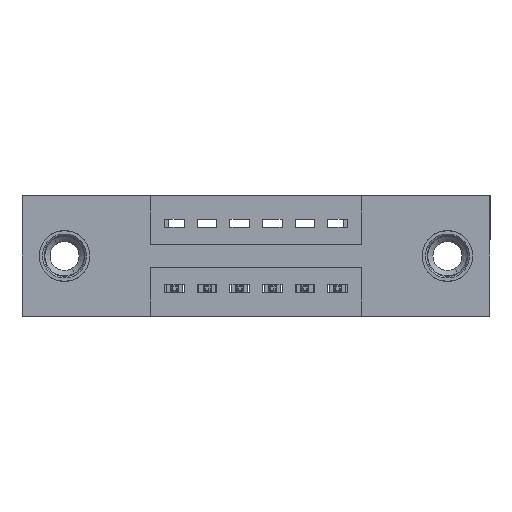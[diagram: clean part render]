
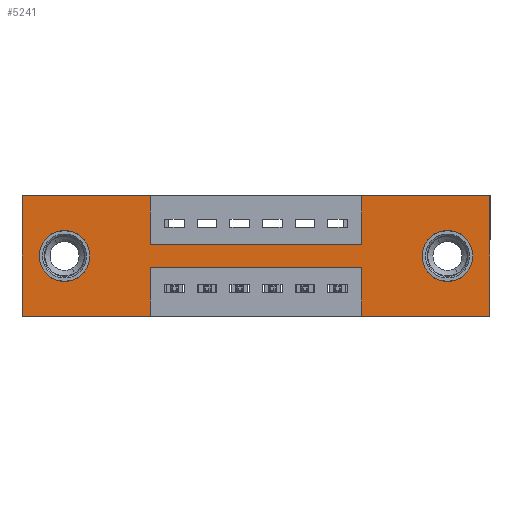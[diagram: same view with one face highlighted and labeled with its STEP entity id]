
A CAD part, front view. The second image highlights one B-rep face of the part: STEP entity #5241.
In plain terms, the highlighted planar face has unit normal (0, -1, 0).
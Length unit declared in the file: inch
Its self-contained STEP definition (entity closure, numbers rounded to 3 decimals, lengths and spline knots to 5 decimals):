
#17 = VECTOR ( 'NONE', #4863, 39.37008 ) ;
#43 = FACE_BOUND ( 'NONE', #11354, .T. ) ;
#104 = CARTESIAN_POINT ( 'NONE',  ( 0., 0., 0. ) ) ;
#146 = LINE ( 'NONE', #10268, #17 ) ;
#180 = FACE_BOUND ( 'NONE', #6715, .T. ) ;
#219 = LINE ( 'NONE', #3082, #7066 ) ;
#233 = CIRCLE ( 'NONE', #9413, 0.078 ) ;
#459 = CARTESIAN_POINT ( 'NONE',  ( 0.3925, 0., -0.37 ) ) ;
#470 = EDGE_CURVE ( 'NONE', #2482, #10637, #7007, .T. ) ;
#523 = ORIENTED_EDGE ( 'NONE', *, *, #9056, .F. ) ;
#635 = DIRECTION ( 'NONE',  ( 0., 0., 1. ) ) ;
#657 = VECTOR ( 'NONE', #8724, 39.37008 ) ;
#661 = EDGE_CURVE ( 'NONE', #3504, #2567, #8666, .T. ) ;
#708 = CARTESIAN_POINT ( 'NONE',  ( 0.13, 0., -0.185 ) ) ;
#1033 = EDGE_CURVE ( 'NONE', #4580, #10286, #233, .T. ) ;
#1054 = ORIENTED_EDGE ( 'NONE', *, *, #7691, .F. ) ;
#1228 = VECTOR ( 'NONE', #2541, 39.37008 ) ;
#1358 = CARTESIAN_POINT ( 'NONE',  ( 1.0425, 0., -0.37 ) ) ;
#1514 = DIRECTION ( 'NONE',  ( 0., 0., 1. ) ) ;
#1562 = EDGE_CURVE ( 'NONE', #10637, #1788, #7770, .T. ) ;
#1593 = VERTEX_POINT ( 'NONE', #459 ) ;
#1699 = EDGE_CURVE ( 'NONE', #10286, #4580, #2029, .T. ) ;
#1788 = VERTEX_POINT ( 'NONE', #7970 ) ;
#1965 = CARTESIAN_POINT ( 'NONE',  ( 0., 0., 0. ) ) ;
#2029 = CIRCLE ( 'NONE', #9501, 0.078 ) ;
#2146 = AXIS2_PLACEMENT_3D ( 'NONE', #708, #7070, #7958 ) ;
#2389 = CARTESIAN_POINT ( 'NONE',  ( 1.0425, 0., -0.37 ) ) ;
#2407 = DIRECTION ( 'NONE',  ( 0., 1., 0. ) ) ;
#2482 = VERTEX_POINT ( 'NONE', #2389 ) ;
#2541 = DIRECTION ( 'NONE',  ( 1., 0., 0. ) ) ;
#2544 = ORIENTED_EDGE ( 'NONE', *, *, #1699, .T. ) ;
#2567 = VERTEX_POINT ( 'NONE', #7847 ) ;
#2642 = VERTEX_POINT ( 'NONE', #10920 ) ;
#2675 = EDGE_CURVE ( 'NONE', #8508, #5809, #8761, .T. ) ;
#2683 = EDGE_CURVE ( 'NONE', #10607, #2482, #9181, .T. ) ;
#2784 = CARTESIAN_POINT ( 'NONE',  ( 0.3925, 0., 0. ) ) ;
#2959 = VERTEX_POINT ( 'NONE', #7315 ) ;
#3060 = LINE ( 'NONE', #6096, #1228 ) ;
#3082 = CARTESIAN_POINT ( 'NONE',  ( 0., 0., -0.37 ) ) ;
#3103 = ORIENTED_EDGE ( 'NONE', *, *, #1562, .F. ) ;
#3242 = VECTOR ( 'NONE', #1514, 39.37008 ) ;
#3504 = VERTEX_POINT ( 'NONE', #9327 ) ;
#3509 = AXIS2_PLACEMENT_3D ( 'NONE', #11296, #5954, #635 ) ;
#3609 = DIRECTION ( 'NONE',  ( 0., 0., -1. ) ) ;
#3691 = EDGE_CURVE ( 'NONE', #10549, #3504, #5065, .T. ) ;
#3826 = VERTEX_POINT ( 'NONE', #5924 ) ;
#4107 = CARTESIAN_POINT ( 'NONE',  ( 0.13, 0., -0.107 ) ) ;
#4234 = PLANE ( 'NONE',  #11470 ) ;
#4265 = ORIENTED_EDGE ( 'NONE', *, *, #4468, .T. ) ;
#4450 = CIRCLE ( 'NONE', #2146, 0.078 ) ;
#4468 = EDGE_CURVE ( 'NONE', #5205, #2642, #8943, .T. ) ;
#4569 = EDGE_CURVE ( 'NONE', #2642, #5205, #4450, .T. ) ;
#4580 = VERTEX_POINT ( 'NONE', #11513 ) ;
#4613 = EDGE_CURVE ( 'NONE', #2959, #3826, #3060, .T. ) ;
#4863 = DIRECTION ( 'NONE',  ( 1., 0., 0. ) ) ;
#5064 = DIRECTION ( 'NONE',  ( 0., -1., 0. ) ) ;
#5065 = LINE ( 'NONE', #2784, #7157 ) ;
#5131 = EDGE_LOOP ( 'NONE', ( #523, #3103, #6701, #5270, #8133, #9442, #1054, #9824, #9307, #5252, #9196, #10583 ) ) ;
#5167 = CARTESIAN_POINT ( 'NONE',  ( 1.0425, 0., 0. ) ) ;
#5205 = VERTEX_POINT ( 'NONE', #4107 ) ;
#5231 = LINE ( 'NONE', #5251, #8160 ) ;
#5241 = ADVANCED_FACE ( 'NONE', ( #43, #180, #6618 ), #4234, .T. ) ;
#5251 = CARTESIAN_POINT ( 'NONE',  ( 0.3925, 0., -0.37 ) ) ;
#5252 = ORIENTED_EDGE ( 'NONE', *, *, #10507, .F. ) ;
#5270 = ORIENTED_EDGE ( 'NONE', *, *, #2683, .F. ) ;
#5283 = DIRECTION ( 'NONE',  ( 0., 0., -1. ) ) ;
#5401 = DIRECTION ( 'NONE',  ( -1., 0., 0. ) ) ;
#5557 = DIRECTION ( 'NONE',  ( 0., 0., 1. ) ) ;
#5809 = VERTEX_POINT ( 'NONE', #1965 ) ;
#5924 = CARTESIAN_POINT ( 'NONE',  ( 1.435, 0., 0. ) ) ;
#5954 = DIRECTION ( 'NONE',  ( 0., 1., 0. ) ) ;
#6096 = CARTESIAN_POINT ( 'NONE',  ( 0., 0., 0. ) ) ;
#6148 = VECTOR ( 'NONE', #9703, 39.37008 ) ;
#6312 = CARTESIAN_POINT ( 'NONE',  ( 0., 0., -0.37 ) ) ;
#6618 = FACE_OUTER_BOUND ( 'NONE', #5131, .T. ) ;
#6655 = VECTOR ( 'NONE', #5401, 39.37008 ) ;
#6701 = ORIENTED_EDGE ( 'NONE', *, *, #470, .F. ) ;
#6715 = EDGE_LOOP ( 'NONE', ( #4265, #6890 ) ) ;
#6769 = ORIENTED_EDGE ( 'NONE', *, *, #1033, .T. ) ;
#6890 = ORIENTED_EDGE ( 'NONE', *, *, #4569, .T. ) ;
#7007 = LINE ( 'NONE', #1358, #3242 ) ;
#7066 = VECTOR ( 'NONE', #11036, 39.37008 ) ;
#7070 = DIRECTION ( 'NONE',  ( 0., 1., 0. ) ) ;
#7157 = VECTOR ( 'NONE', #3609, 39.37008 ) ;
#7315 = CARTESIAN_POINT ( 'NONE',  ( 1.0425, 0., 0. ) ) ;
#7471 = DIRECTION ( 'NONE',  ( 0., 0., -1. ) ) ;
#7576 = CARTESIAN_POINT ( 'NONE',  ( 1.435, 0., -0.37 ) ) ;
#7669 = CARTESIAN_POINT ( 'NONE',  ( 1.305, 0., -0.263 ) ) ;
#7691 = EDGE_CURVE ( 'NONE', #2567, #2959, #10335, .T. ) ;
#7757 = CARTESIAN_POINT ( 'NONE',  ( 1.305, 0., -0.185 ) ) ;
#7770 = LINE ( 'NONE', #9253, #11003 ) ;
#7847 = CARTESIAN_POINT ( 'NONE',  ( 1.0425, 0., -0.15 ) ) ;
#7903 = VECTOR ( 'NONE', #5557, 39.37008 ) ;
#7958 = DIRECTION ( 'NONE',  ( 0., 0., 1. ) ) ;
#7969 = VECTOR ( 'NONE', #9536, 39.37008 ) ;
#7970 = CARTESIAN_POINT ( 'NONE',  ( 0.3925, 0., -0.22 ) ) ;
#8133 = ORIENTED_EDGE ( 'NONE', *, *, #10590, .F. ) ;
#8160 = VECTOR ( 'NONE', #5283, 39.37008 ) ;
#8225 = EDGE_CURVE ( 'NONE', #1593, #8508, #219, .T. ) ;
#8465 = DIRECTION ( 'NONE',  ( 0., 1., 0. ) ) ;
#8508 = VERTEX_POINT ( 'NONE', #11133 ) ;
#8606 = DIRECTION ( 'NONE',  ( 0., 0., -1. ) ) ;
#8666 = LINE ( 'NONE', #9631, #6148 ) ;
#8724 = DIRECTION ( 'NONE',  ( 0., 0., 1. ) ) ;
#8761 = LINE ( 'NONE', #104, #7903 ) ;
#8876 = CARTESIAN_POINT ( 'NONE',  ( 1.0425, 0., -0.22 ) ) ;
#8943 = CIRCLE ( 'NONE', #3509, 0.078 ) ;
#9056 = EDGE_CURVE ( 'NONE', #1788, #1593, #5231, .T. ) ;
#9181 = LINE ( 'NONE', #6312, #6655 ) ;
#9196 = ORIENTED_EDGE ( 'NONE', *, *, #2675, .F. ) ;
#9253 = CARTESIAN_POINT ( 'NONE',  ( 0.3925, 0., -0.22 ) ) ;
#9307 = ORIENTED_EDGE ( 'NONE', *, *, #3691, .F. ) ;
#9327 = CARTESIAN_POINT ( 'NONE',  ( 0.3925, 0., -0.15 ) ) ;
#9413 = AXIS2_PLACEMENT_3D ( 'NONE', #10293, #8465, #7471 ) ;
#9442 = ORIENTED_EDGE ( 'NONE', *, *, #4613, .F. ) ;
#9501 = AXIS2_PLACEMENT_3D ( 'NONE', #7757, #2407, #9577 ) ;
#9536 = DIRECTION ( 'NONE',  ( 0., 0., -1. ) ) ;
#9575 = CARTESIAN_POINT ( 'NONE',  ( 1.435, 0., 0. ) ) ;
#9577 = DIRECTION ( 'NONE',  ( 0., 0., -1. ) ) ;
#9631 = CARTESIAN_POINT ( 'NONE',  ( 0.3925, 0., -0.15 ) ) ;
#9703 = DIRECTION ( 'NONE',  ( 1., 0., 0. ) ) ;
#9824 = ORIENTED_EDGE ( 'NONE', *, *, #661, .F. ) ;
#9829 = LINE ( 'NONE', #9575, #7969 ) ;
#10231 = CARTESIAN_POINT ( 'NONE',  ( 0.3925, 0., 0. ) ) ;
#10234 = DIRECTION ( 'NONE',  ( -1., 0., 0. ) ) ;
#10268 = CARTESIAN_POINT ( 'NONE',  ( 0., 0., 0. ) ) ;
#10286 = VERTEX_POINT ( 'NONE', #7669 ) ;
#10293 = CARTESIAN_POINT ( 'NONE',  ( 1.305, 0., -0.185 ) ) ;
#10335 = LINE ( 'NONE', #5167, #657 ) ;
#10504 = CARTESIAN_POINT ( 'NONE',  ( 0., 0., -0.37 ) ) ;
#10507 = EDGE_CURVE ( 'NONE', #5809, #10549, #146, .T. ) ;
#10549 = VERTEX_POINT ( 'NONE', #10231 ) ;
#10583 = ORIENTED_EDGE ( 'NONE', *, *, #8225, .F. ) ;
#10590 = EDGE_CURVE ( 'NONE', #3826, #10607, #9829, .T. ) ;
#10607 = VERTEX_POINT ( 'NONE', #7576 ) ;
#10637 = VERTEX_POINT ( 'NONE', #8876 ) ;
#10920 = CARTESIAN_POINT ( 'NONE',  ( 0.13, 0., -0.263 ) ) ;
#11003 = VECTOR ( 'NONE', #10234, 39.37008 ) ;
#11036 = DIRECTION ( 'NONE',  ( -1., 0., 0. ) ) ;
#11133 = CARTESIAN_POINT ( 'NONE',  ( 0., 0., -0.37 ) ) ;
#11296 = CARTESIAN_POINT ( 'NONE',  ( 0.13, 0., -0.185 ) ) ;
#11354 = EDGE_LOOP ( 'NONE', ( #6769, #2544 ) ) ;
#11470 = AXIS2_PLACEMENT_3D ( 'NONE', #10504, #5064, #8606 ) ;
#11513 = CARTESIAN_POINT ( 'NONE',  ( 1.305, 0., -0.107 ) ) ;
